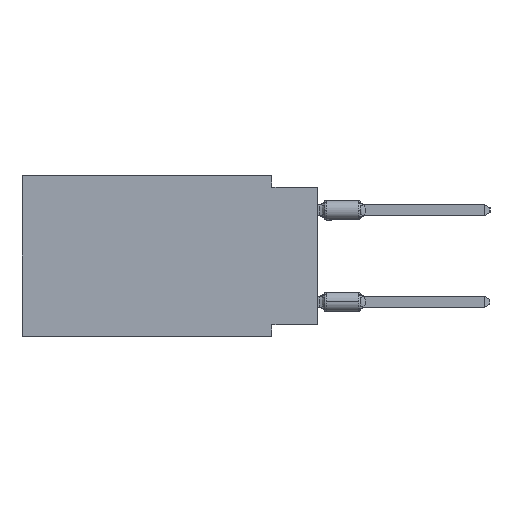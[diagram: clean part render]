
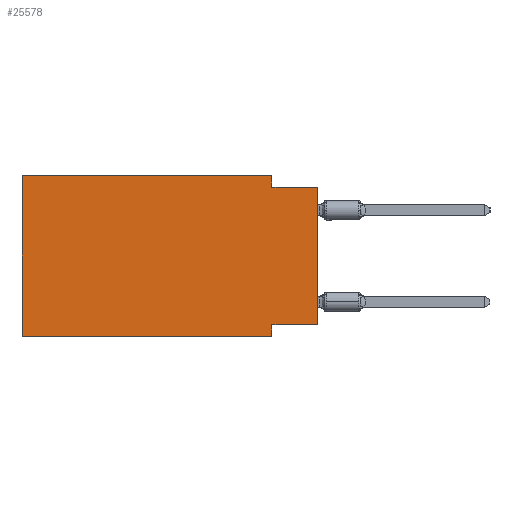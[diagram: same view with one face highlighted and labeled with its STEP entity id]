
A CAD part, left-side view. The second image highlights one B-rep face of the part: STEP entity #25578.
In plain terms, the highlighted planar face has unit normal (-1, 0, 0).
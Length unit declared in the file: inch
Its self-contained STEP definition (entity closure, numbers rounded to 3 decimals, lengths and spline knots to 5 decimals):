
#1315 = DIRECTION ( 'NONE',  ( 0., -1., 0. ) ) ;
#3632 = ORIENTED_EDGE ( 'NONE', *, *, #49006, .F. ) ;
#3775 = VECTOR ( 'NONE', #50970, 39.37008 ) ;
#4699 = EDGE_CURVE ( 'NONE', #7190, #34980, #41405, .T. ) ;
#4961 = DIRECTION ( 'NONE',  ( 0., -1., 0. ) ) ;
#5525 = EDGE_CURVE ( 'NONE', #48064, #36010, #8537, .T. ) ;
#5549 = EDGE_CURVE ( 'NONE', #48064, #32690, #27668, .T. ) ;
#6648 = LINE ( 'NONE', #49854, #21675 ) ;
#6693 = ORIENTED_EDGE ( 'NONE', *, *, #4699, .F. ) ;
#7190 = VERTEX_POINT ( 'NONE', #59206 ) ;
#8424 = PLANE ( 'NONE',  #56597 ) ;
#8537 = LINE ( 'NONE', #22132, #28754 ) ;
#8590 = EDGE_CURVE ( 'NONE', #32690, #56286, #49459, .T. ) ;
#9739 = VECTOR ( 'NONE', #4961, 39.37008 ) ;
#10101 = CARTESIAN_POINT ( 'NONE',  ( 0., 0., -0.325 ) ) ;
#10898 = VERTEX_POINT ( 'NONE', #50607 ) ;
#11077 = CARTESIAN_POINT ( 'NONE',  ( 0., 0., -0.025 ) ) ;
#12875 = DIRECTION ( 'NONE',  ( 0., 1., 0. ) ) ;
#14662 = EDGE_CURVE ( 'NONE', #10898, #56286, #33041, .T. ) ;
#15782 = CARTESIAN_POINT ( 'NONE',  ( 0., 0.645, 0. ) ) ;
#17120 = ORIENTED_EDGE ( 'NONE', *, *, #8590, .F. ) ;
#18007 = DIRECTION ( 'NONE',  ( 0., 0., -1. ) ) ;
#18147 = CARTESIAN_POINT ( 'NONE',  ( 0., 0.645, 0. ) ) ;
#18401 = DIRECTION ( 'NONE',  ( 0., 0., 1. ) ) ;
#20820 = ORIENTED_EDGE ( 'NONE', *, *, #14662, .T. ) ;
#21675 = VECTOR ( 'NONE', #43988, 39.37008 ) ;
#21985 = CARTESIAN_POINT ( 'NONE',  ( 0., 0.1, -0.35 ) ) ;
#22132 = CARTESIAN_POINT ( 'NONE',  ( 0., 0., 0. ) ) ;
#22950 = VERTEX_POINT ( 'NONE', #18147 ) ;
#23230 = ORIENTED_EDGE ( 'NONE', *, *, #5549, .F. ) ;
#23484 = CARTESIAN_POINT ( 'NONE',  ( 0., 0.645, -0.35 ) ) ;
#24058 = EDGE_LOOP ( 'NONE', ( #47528, #56147, #6693, #3632, #55981, #20820, #17120, #23230 ) ) ;
#25249 = EDGE_CURVE ( 'NONE', #10898, #22950, #33490, .T. ) ;
#25578 = ADVANCED_FACE ( 'NONE', ( #45766 ), #8424, .F. ) ;
#27668 = LINE ( 'NONE', #61027, #59351 ) ;
#28754 = VECTOR ( 'NONE', #18401, 39.37008 ) ;
#28856 = DIRECTION ( 'NONE',  ( 0., 0., 1. ) ) ;
#31172 = CARTESIAN_POINT ( 'NONE',  ( 0., 0.1, -0.35 ) ) ;
#32690 = VERTEX_POINT ( 'NONE', #47348 ) ;
#33041 = LINE ( 'NONE', #23484, #9739 ) ;
#33490 = LINE ( 'NONE', #47374, #38822 ) ;
#34980 = VERTEX_POINT ( 'NONE', #36954 ) ;
#36010 = VERTEX_POINT ( 'NONE', #11077 ) ;
#36954 = CARTESIAN_POINT ( 'NONE',  ( 0., 0.1, -0.025 ) ) ;
#38822 = VECTOR ( 'NONE', #28856, 39.37008 ) ;
#39520 = VECTOR ( 'NONE', #39880, 39.37008 ) ;
#39719 = EDGE_CURVE ( 'NONE', #34980, #36010, #6648, .T. ) ;
#39880 = DIRECTION ( 'NONE',  ( 0., 0., -1. ) ) ;
#41405 = LINE ( 'NONE', #60264, #3775 ) ;
#43856 = LINE ( 'NONE', #15782, #47080 ) ;
#43988 = DIRECTION ( 'NONE',  ( 0., -1., 0. ) ) ;
#45160 = CARTESIAN_POINT ( 'NONE',  ( 0., 0.645, 0. ) ) ;
#45766 = FACE_OUTER_BOUND ( 'NONE', #24058, .T. ) ;
#47080 = VECTOR ( 'NONE', #1315, 39.37008 ) ;
#47348 = CARTESIAN_POINT ( 'NONE',  ( 0., 0.1, -0.325 ) ) ;
#47374 = CARTESIAN_POINT ( 'NONE',  ( 0., 0.645, 0. ) ) ;
#47528 = ORIENTED_EDGE ( 'NONE', *, *, #5525, .T. ) ;
#48064 = VERTEX_POINT ( 'NONE', #10101 ) ;
#49006 = EDGE_CURVE ( 'NONE', #22950, #7190, #43856, .T. ) ;
#49459 = LINE ( 'NONE', #21985, #39520 ) ;
#49854 = CARTESIAN_POINT ( 'NONE',  ( 0., 0., -0.025 ) ) ;
#50607 = CARTESIAN_POINT ( 'NONE',  ( 0., 0.645, -0.35 ) ) ;
#50970 = DIRECTION ( 'NONE',  ( 0., 0., -1. ) ) ;
#55357 = DIRECTION ( 'NONE',  ( 1., 0., 0. ) ) ;
#55981 = ORIENTED_EDGE ( 'NONE', *, *, #25249, .F. ) ;
#56147 = ORIENTED_EDGE ( 'NONE', *, *, #39719, .F. ) ;
#56286 = VERTEX_POINT ( 'NONE', #31172 ) ;
#56597 = AXIS2_PLACEMENT_3D ( 'NONE', #45160, #55357, #18007 ) ;
#59206 = CARTESIAN_POINT ( 'NONE',  ( 0., 0.1, 0. ) ) ;
#59351 = VECTOR ( 'NONE', #12875, 39.37008 ) ;
#60264 = CARTESIAN_POINT ( 'NONE',  ( 0., 0.1, 0. ) ) ;
#61027 = CARTESIAN_POINT ( 'NONE',  ( 0., 0., -0.325 ) ) ;
